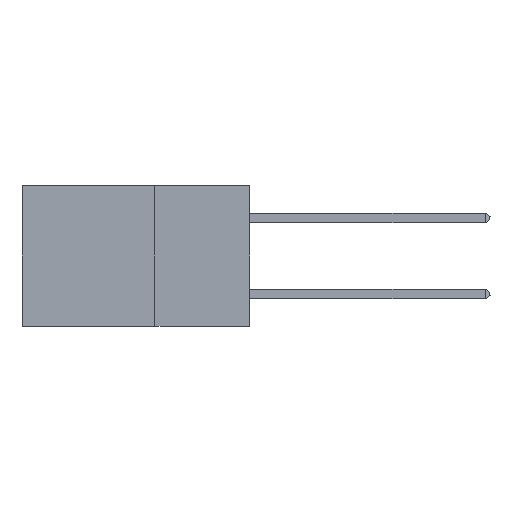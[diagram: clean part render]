
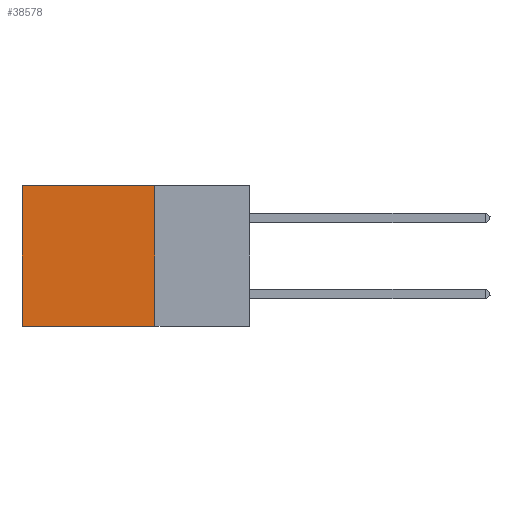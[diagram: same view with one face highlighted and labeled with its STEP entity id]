
A CAD part, left-side view. The second image highlights one B-rep face of the part: STEP entity #38578.
In plain terms, the highlighted planar face has unit normal (-1, 0, 0).
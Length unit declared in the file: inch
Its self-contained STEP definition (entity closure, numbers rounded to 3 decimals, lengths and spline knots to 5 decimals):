
#39 = DIRECTION ( 'NONE',  ( 0., 0., -1. ) ) ;
#1515 = CARTESIAN_POINT ( 'NONE',  ( 0.2875, 0.25, 0. ) ) ;
#1569 = DIRECTION ( 'NONE',  ( 1., 0., 0. ) ) ;
#1957 = LINE ( 'NONE', #25624, #38450 ) ;
#2835 = CARTESIAN_POINT ( 'NONE',  ( 0.2875, 0.25, 0. ) ) ;
#3330 = LINE ( 'NONE', #18387, #33697 ) ;
#3808 = EDGE_CURVE ( 'NONE', #30366, #22209, #12071, .T. ) ;
#7233 = EDGE_CURVE ( 'NONE', #35323, #17882, #3330, .T. ) ;
#9920 = CARTESIAN_POINT ( 'NONE',  ( 0.2875, 0.6, 0. ) ) ;
#10595 = DIRECTION ( 'NONE',  ( 0., 0., -1. ) ) ;
#12071 = LINE ( 'NONE', #2835, #14389 ) ;
#14389 = VECTOR ( 'NONE', #23899, 39.37008 ) ;
#17882 = VERTEX_POINT ( 'NONE', #29437 ) ;
#18387 = CARTESIAN_POINT ( 'NONE',  ( 0.2875, 0.6, 0. ) ) ;
#19476 = CARTESIAN_POINT ( 'NONE',  ( 0.2875, 0.25, 0. ) ) ;
#19529 = ORIENTED_EDGE ( 'NONE', *, *, #26973, .F. ) ;
#20502 = EDGE_LOOP ( 'NONE', ( #23566, #19529, #26384, #35624 ) ) ;
#22209 = VERTEX_POINT ( 'NONE', #35543 ) ;
#23566 = ORIENTED_EDGE ( 'NONE', *, *, #7233, .T. ) ;
#23899 = DIRECTION ( 'NONE',  ( 0., 0., -1. ) ) ;
#25624 = CARTESIAN_POINT ( 'NONE',  ( 0.2875, 0.25, -0.37 ) ) ;
#26384 = ORIENTED_EDGE ( 'NONE', *, *, #3808, .F. ) ;
#26973 = EDGE_CURVE ( 'NONE', #22209, #17882, #1957, .T. ) ;
#28336 = CARTESIAN_POINT ( 'NONE',  ( 0.2875, 0.25, 0. ) ) ;
#28360 = DIRECTION ( 'NONE',  ( 0., 1., 0. ) ) ;
#29437 = CARTESIAN_POINT ( 'NONE',  ( 0.2875, 0.6, -0.37 ) ) ;
#30159 = VECTOR ( 'NONE', #37703, 39.37008 ) ;
#30366 = VERTEX_POINT ( 'NONE', #1515 ) ;
#32041 = LINE ( 'NONE', #28336, #30159 ) ;
#33697 = VECTOR ( 'NONE', #39, 39.37008 ) ;
#34413 = EDGE_CURVE ( 'NONE', #30366, #35323, #32041, .T. ) ;
#35323 = VERTEX_POINT ( 'NONE', #9920 ) ;
#35543 = CARTESIAN_POINT ( 'NONE',  ( 0.2875, 0.25, -0.37 ) ) ;
#35624 = ORIENTED_EDGE ( 'NONE', *, *, #34413, .T. ) ;
#36908 = FACE_OUTER_BOUND ( 'NONE', #20502, .T. ) ;
#37334 = PLANE ( 'NONE',  #38360 ) ;
#37703 = DIRECTION ( 'NONE',  ( 0., 1., 0. ) ) ;
#38360 = AXIS2_PLACEMENT_3D ( 'NONE', #19476, #1569, #10595 ) ;
#38450 = VECTOR ( 'NONE', #28360, 39.37008 ) ;
#38578 = ADVANCED_FACE ( 'NONE', ( #36908 ), #37334, .F. ) ;
